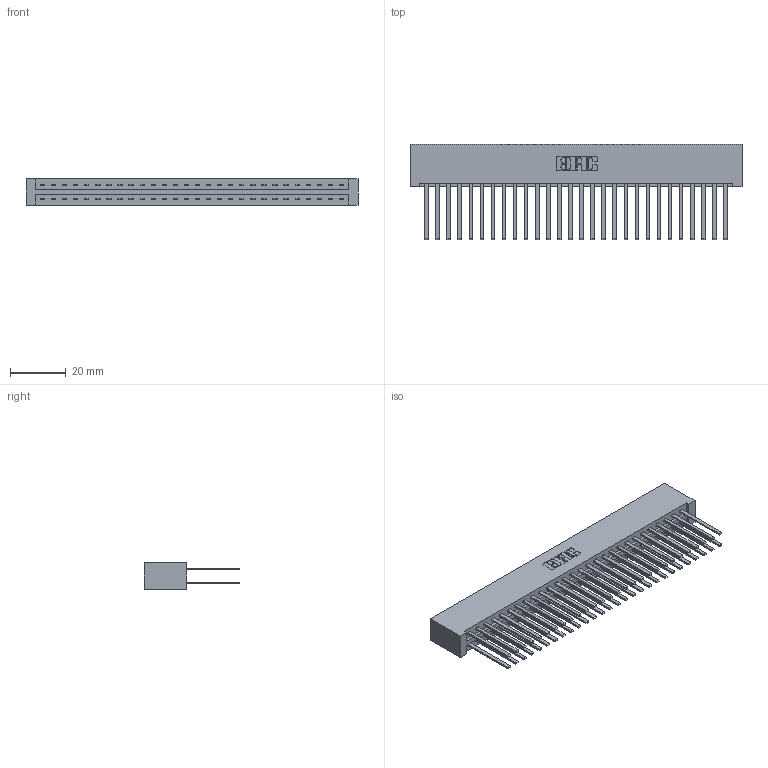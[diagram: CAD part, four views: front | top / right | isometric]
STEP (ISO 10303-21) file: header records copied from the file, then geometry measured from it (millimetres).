
FILE_DESCRIPTION (( 'STEP AP203' ), '1' );
FILE_NAME ('387-056-544-201.STEP', '2019-10-19T07:15:17', ( '' ), ( '' ), 'SwSTEP 2.0', 'SolidWorks 2016', '' );
FILE_SCHEMA (( 'CONFIG_CONTROL_DESIGN' ));
Length unit declared in the file: inch
Products named in the file (3): 345-292-001_345-293-144; 387-056-544-201; 337 Part_No Mounting Lugs
Assembly tree (57 placements, depth 2):
  387-056-544-201
    337 Part_No Mounting Lugs
    345-292-001_345-293-144  x56
Bounding box: 118.82 x 34.3 x 9.4 mm (x, y, z)
Volume: 13881.7 mm3; surface area: 18177.9 mm2
Topology: 57 solids, 57 shells, 2794 faces, 8295 edges, 5454 vertices
Faces by surface type: plane 1970, cylinder 824
Entity records: 23059 total; most frequent: CARTESIAN_POINT 3894, ORIENTED_EDGE 3830, DIRECTION 3327, EDGE_CURVE 1915, VECTOR 1799, LINE 1799, VERTEX_POINT 1274, AXIS2_PLACEMENT_3D 764
